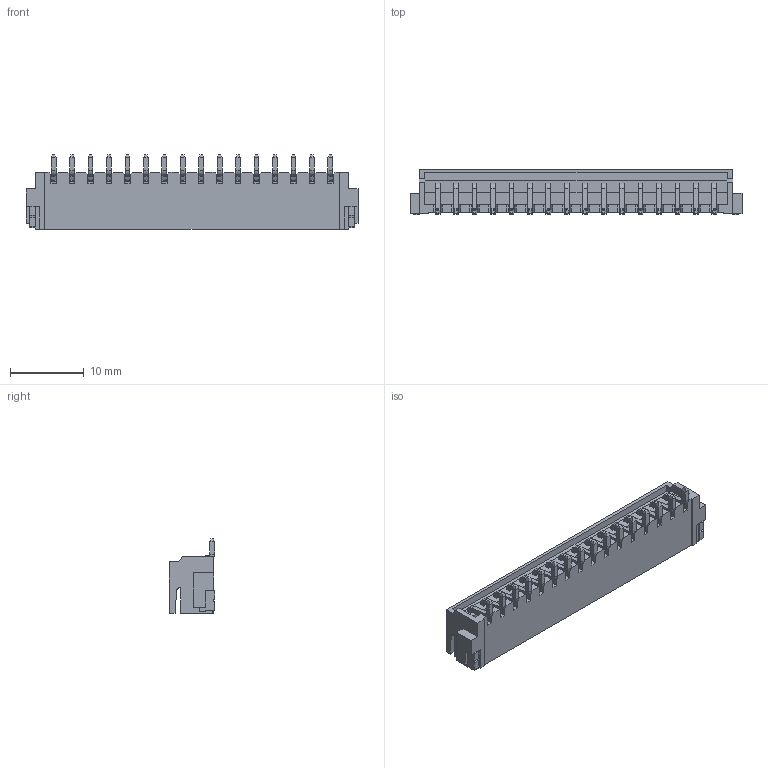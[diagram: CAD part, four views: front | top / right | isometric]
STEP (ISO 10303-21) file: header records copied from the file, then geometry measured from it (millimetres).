
FILE_DESCRIPTION (( 'STEP AP203' ), '1' );
FILE_NAME ('14K-516-418TAA1.STEP', '2024-02-22T13:39:56', ( '' ), ( '' ), 'SwSTEP 2.0', 'SolidWorks 2023', '' );
FILE_SCHEMA (( 'CONFIG_CONTROL_DESIGN' ));
Length unit declared in the file: millimetre
Products named in the file (3): 14K-516-418TAA1; 14K Series SMT Pin_Side Entry; 14K Series SMT Side Entry Insulator_516
Assembly tree (17 placements, depth 2):
  14K-516-418TAA1
    14K Series SMT Side Entry Insulator_516
    14K Series SMT Pin_Side Entry  x16
Bounding box: 45 x 6.1 x 10.15 mm (x, y, z)
Volume: 774.9 mm3; surface area: 2514.7 mm2
Topology: 17 solids, 17 shells, 917 faces, 2225 edges, 1342 vertices
Faces by surface type: plane 814, cylinder 103
Entity records: 14692 total; most frequent: CARTESIAN_POINT 2494, ORIENTED_EDGE 2470, DIRECTION 2235, EDGE_CURVE 1235, LINE 1149, VECTOR 1149, VERTEX_POINT 802, AXIS2_PLACEMENT_3D 543
